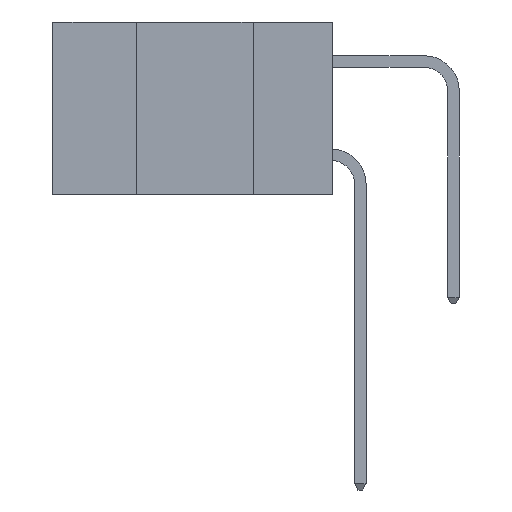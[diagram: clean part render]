
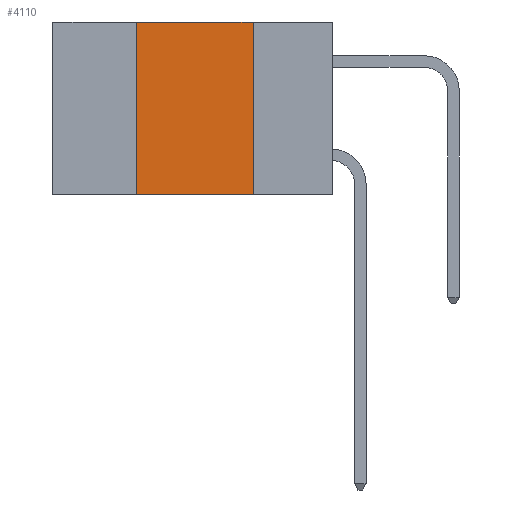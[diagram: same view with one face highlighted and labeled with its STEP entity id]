
A CAD part, left-side view. The second image highlights one B-rep face of the part: STEP entity #4110.
In plain terms, the highlighted planar face has unit normal (-1, 0, 0).
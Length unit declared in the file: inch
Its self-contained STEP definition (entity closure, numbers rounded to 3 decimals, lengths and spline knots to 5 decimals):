
#429 = DIRECTION ( 'NONE',  ( 0., 0., -1. ) ) ;
#536 = CARTESIAN_POINT ( 'NONE',  ( 0., 0.17, -0.37 ) ) ;
#1017 = VECTOR ( 'NONE', #5082, 39.37008 ) ;
#1197 = VERTEX_POINT ( 'NONE', #1670 ) ;
#1293 = VERTEX_POINT ( 'NONE', #6051 ) ;
#1670 = CARTESIAN_POINT ( 'NONE',  ( 0., 0.17, 0. ) ) ;
#2368 = CARTESIAN_POINT ( 'NONE',  ( 0., 0.42, -0.37 ) ) ;
#2381 = DIRECTION ( 'NONE',  ( 0., 0., -1. ) ) ;
#2692 = VERTEX_POINT ( 'NONE', #9993 ) ;
#3024 = VECTOR ( 'NONE', #7744, 39.37008 ) ;
#3299 = FACE_OUTER_BOUND ( 'NONE', #7541, .T. ) ;
#3370 = DIRECTION ( 'NONE',  ( 0., -1., 0. ) ) ;
#3435 = LINE ( 'NONE', #8696, #1017 ) ;
#4038 = CARTESIAN_POINT ( 'NONE',  ( 0., 0.6, 0. ) ) ;
#4109 = VECTOR ( 'NONE', #2381, 39.37008 ) ;
#4110 = ADVANCED_FACE ( 'NONE', ( #3299 ), #11181, .F. ) ;
#5082 = DIRECTION ( 'NONE',  ( 0., -1., 0. ) ) ;
#5108 = VERTEX_POINT ( 'NONE', #7331 ) ;
#5810 = DIRECTION ( 'NONE',  ( 1., 0., 0. ) ) ;
#6051 = CARTESIAN_POINT ( 'NONE',  ( 0., 0.42, 0. ) ) ;
#6494 = LINE ( 'NONE', #536, #4109 ) ;
#6701 = ORIENTED_EDGE ( 'NONE', *, *, #9103, .F. ) ;
#6986 = ORIENTED_EDGE ( 'NONE', *, *, #7896, .F. ) ;
#7270 = ORIENTED_EDGE ( 'NONE', *, *, #7296, .T. ) ;
#7296 = EDGE_CURVE ( 'NONE', #5108, #2692, #11561, .T. ) ;
#7331 = CARTESIAN_POINT ( 'NONE',  ( 0., 0.42, -0.37 ) ) ;
#7391 = VECTOR ( 'NONE', #3370, 39.37008 ) ;
#7541 = EDGE_LOOP ( 'NONE', ( #6701, #9099, #6986, #7270 ) ) ;
#7744 = DIRECTION ( 'NONE',  ( 0., 0., 1. ) ) ;
#7896 = EDGE_CURVE ( 'NONE', #5108, #1293, #10181, .T. ) ;
#7954 = AXIS2_PLACEMENT_3D ( 'NONE', #4038, #5810, #429 ) ;
#8513 = EDGE_CURVE ( 'NONE', #1293, #1197, #3435, .T. ) ;
#8696 = CARTESIAN_POINT ( 'NONE',  ( 0., 0.6, 0. ) ) ;
#8758 = CARTESIAN_POINT ( 'NONE',  ( 0., 0.6, -0.37 ) ) ;
#9099 = ORIENTED_EDGE ( 'NONE', *, *, #8513, .F. ) ;
#9103 = EDGE_CURVE ( 'NONE', #1197, #2692, #6494, .T. ) ;
#9993 = CARTESIAN_POINT ( 'NONE',  ( 0., 0.17, -0.37 ) ) ;
#10181 = LINE ( 'NONE', #2368, #3024 ) ;
#11181 = PLANE ( 'NONE',  #7954 ) ;
#11561 = LINE ( 'NONE', #8758, #7391 ) ;
